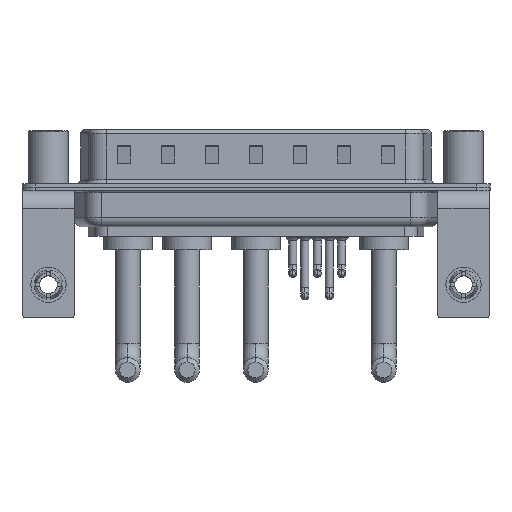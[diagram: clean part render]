
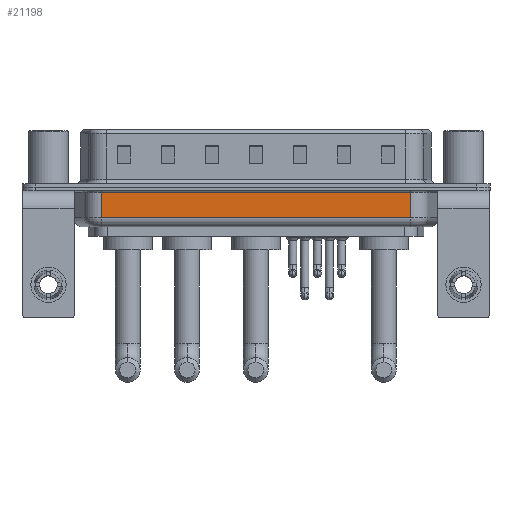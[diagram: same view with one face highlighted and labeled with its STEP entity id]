
A CAD part, front view. The second image highlights one B-rep face of the part: STEP entity #21198.
In plain terms, the highlighted planar face has unit normal (0, -1, 0).
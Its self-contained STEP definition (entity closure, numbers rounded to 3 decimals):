
#453 = VERTEX_POINT ( 'NONE', #12640 ) ;
#1278 = EDGE_CURVE ( 'NONE', #453, #3661, #4005, .T. ) ;
#1641 = DIRECTION ( 'NONE',  ( -1., 0., 0. ) ) ;
#1642 = ORIENTED_EDGE ( 'NONE', *, *, #1278, .T. ) ;
#3295 = CARTESIAN_POINT ( 'NONE',  ( 6.006, -5.35, -3.5 ) ) ;
#3661 = VERTEX_POINT ( 'NONE', #10863 ) ;
#4005 = LINE ( 'NONE', #18300, #20539 ) ;
#4667 = CARTESIAN_POINT ( 'NONE',  ( 6.006, -5.35, -3.5 ) ) ;
#5278 = PLANE ( 'NONE',  #17321 ) ;
#6105 = CARTESIAN_POINT ( 'NONE',  ( 6.006, -5.35, -4.5 ) ) ;
#6498 = DIRECTION ( 'NONE',  ( 0., 0., 1. ) ) ;
#6568 = CARTESIAN_POINT ( 'NONE',  ( 6.006, -5.35, -0.65 ) ) ;
#6734 = ORIENTED_EDGE ( 'NONE', *, *, #25074, .F. ) ;
#9104 = FACE_OUTER_BOUND ( 'NONE', #20308, .T. ) ;
#10863 = CARTESIAN_POINT ( 'NONE',  ( 41.044, -5.35, -0.65 ) ) ;
#11224 = EDGE_CURVE ( 'NONE', #3661, #12457, #21624, .T. ) ;
#11583 = DIRECTION ( 'NONE',  ( 0., 0., 1. ) ) ;
#11838 = DIRECTION ( 'NONE',  ( 1., 0., 0. ) ) ;
#12270 = DIRECTION ( 'NONE',  ( 0., 0., 1. ) ) ;
#12457 = VERTEX_POINT ( 'NONE', #6568 ) ;
#12640 = CARTESIAN_POINT ( 'NONE',  ( 41.044, -5.35, -3.5 ) ) ;
#13193 = DIRECTION ( 'NONE',  ( 0., 1., 0. ) ) ;
#14049 = VECTOR ( 'NONE', #11838, 1000. ) ;
#15700 = CARTESIAN_POINT ( 'NONE',  ( 6.006, -5.35, -0.65 ) ) ;
#17205 = VECTOR ( 'NONE', #1641, 1000. ) ;
#17321 = AXIS2_PLACEMENT_3D ( 'NONE', #19310, #13193, #11583 ) ;
#17843 = VECTOR ( 'NONE', #12270, 1000. ) ;
#18300 = CARTESIAN_POINT ( 'NONE',  ( 41.044, -5.35, -4.5 ) ) ;
#19310 = CARTESIAN_POINT ( 'NONE',  ( 6.006, -5.35, -4.5 ) ) ;
#20308 = EDGE_LOOP ( 'NONE', ( #6734, #25822, #1642, #21845 ) ) ;
#20539 = VECTOR ( 'NONE', #6498, 1000. ) ;
#21182 = VERTEX_POINT ( 'NONE', #3295 ) ;
#21198 = ADVANCED_FACE ( 'NONE', ( #9104 ), #5278, .F. ) ;
#21624 = LINE ( 'NONE', #15700, #17205 ) ;
#21845 = ORIENTED_EDGE ( 'NONE', *, *, #11224, .T. ) ;
#23770 = EDGE_CURVE ( 'NONE', #21182, #453, #23907, .T. ) ;
#23907 = LINE ( 'NONE', #4667, #14049 ) ;
#24089 = LINE ( 'NONE', #6105, #17843 ) ;
#25074 = EDGE_CURVE ( 'NONE', #21182, #12457, #24089, .T. ) ;
#25822 = ORIENTED_EDGE ( 'NONE', *, *, #23770, .T. ) ;
